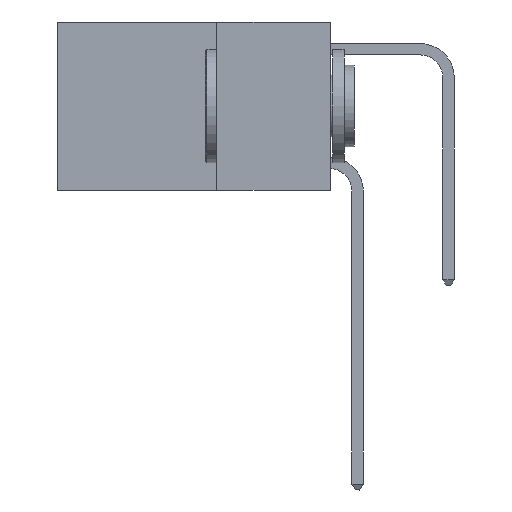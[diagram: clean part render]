
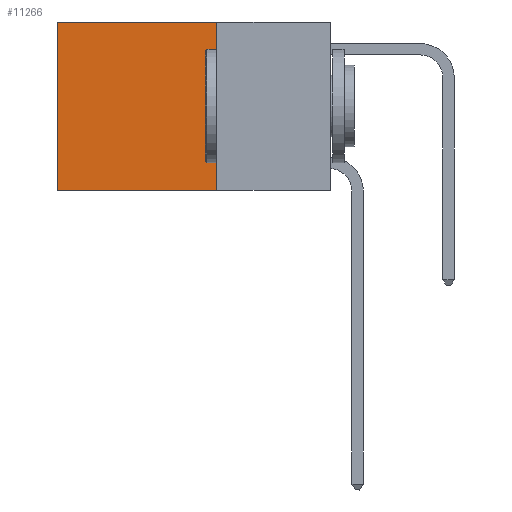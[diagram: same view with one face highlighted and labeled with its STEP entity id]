
A CAD part, left-side view. The second image highlights one B-rep face of the part: STEP entity #11266.
In plain terms, the highlighted planar face has unit normal (-1, 0, 0).
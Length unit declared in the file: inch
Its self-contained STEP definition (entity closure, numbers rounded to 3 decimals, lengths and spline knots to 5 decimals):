
#242 = DIRECTION ( 'NONE',  ( 0., 0., -1. ) ) ;
#296 = ORIENTED_EDGE ( 'NONE', *, *, #11827, .T. ) ;
#571 = DIRECTION ( 'NONE',  ( 0., 1., 0. ) ) ;
#890 = ORIENTED_EDGE ( 'NONE', *, *, #4227, .F. ) ;
#995 = FACE_OUTER_BOUND ( 'NONE', #7009, .T. ) ;
#2307 = ORIENTED_EDGE ( 'NONE', *, *, #6176, .T. ) ;
#3009 = DIRECTION ( 'NONE',  ( 0., 0., -1. ) ) ;
#3775 = LINE ( 'NONE', #7962, #6564 ) ;
#3899 = CARTESIAN_POINT ( 'NONE',  ( 0.2625, 0.6, 0. ) ) ;
#4227 = EDGE_CURVE ( 'NONE', #11625, #9753, #7907, .T. ) ;
#4781 = PLANE ( 'NONE',  #7124 ) ;
#4883 = VECTOR ( 'NONE', #3009, 39.37008 ) ;
#5708 = DIRECTION ( 'NONE',  ( 1., 0., 0. ) ) ;
#6107 = CARTESIAN_POINT ( 'NONE',  ( 0.2625, 0.25, -0.37 ) ) ;
#6176 = EDGE_CURVE ( 'NONE', #7042, #6515, #9690, .T. ) ;
#6483 = CARTESIAN_POINT ( 'NONE',  ( 0.2625, 0.6, 0. ) ) ;
#6515 = VERTEX_POINT ( 'NONE', #6483 ) ;
#6564 = VECTOR ( 'NONE', #242, 39.37008 ) ;
#7009 = EDGE_LOOP ( 'NONE', ( #296, #890, #9586, #2307 ) ) ;
#7042 = VERTEX_POINT ( 'NONE', #10313 ) ;
#7124 = AXIS2_PLACEMENT_3D ( 'NONE', #11403, #5708, #11523 ) ;
#7201 = VECTOR ( 'NONE', #11886, 39.37008 ) ;
#7784 = CARTESIAN_POINT ( 'NONE',  ( 0.2625, 0.25, 0. ) ) ;
#7907 = LINE ( 'NONE', #6107, #12202 ) ;
#7962 = CARTESIAN_POINT ( 'NONE',  ( 0.2625, 0.25, 0. ) ) ;
#8904 = LINE ( 'NONE', #3899, #4883 ) ;
#9147 = EDGE_CURVE ( 'NONE', #7042, #11625, #3775, .T. ) ;
#9586 = ORIENTED_EDGE ( 'NONE', *, *, #9147, .F. ) ;
#9690 = LINE ( 'NONE', #7784, #7201 ) ;
#9753 = VERTEX_POINT ( 'NONE', #11776 ) ;
#10092 = CARTESIAN_POINT ( 'NONE',  ( 0.2625, 0.25, -0.37 ) ) ;
#10313 = CARTESIAN_POINT ( 'NONE',  ( 0.2625, 0.25, 0. ) ) ;
#11266 = ADVANCED_FACE ( 'NONE', ( #995 ), #4781, .F. ) ;
#11403 = CARTESIAN_POINT ( 'NONE',  ( 0.2625, 0.25, 0. ) ) ;
#11523 = DIRECTION ( 'NONE',  ( 0., 0., -1. ) ) ;
#11625 = VERTEX_POINT ( 'NONE', #10092 ) ;
#11776 = CARTESIAN_POINT ( 'NONE',  ( 0.2625, 0.6, -0.37 ) ) ;
#11827 = EDGE_CURVE ( 'NONE', #6515, #9753, #8904, .T. ) ;
#11886 = DIRECTION ( 'NONE',  ( 0., 1., 0. ) ) ;
#12202 = VECTOR ( 'NONE', #571, 39.37008 ) ;
